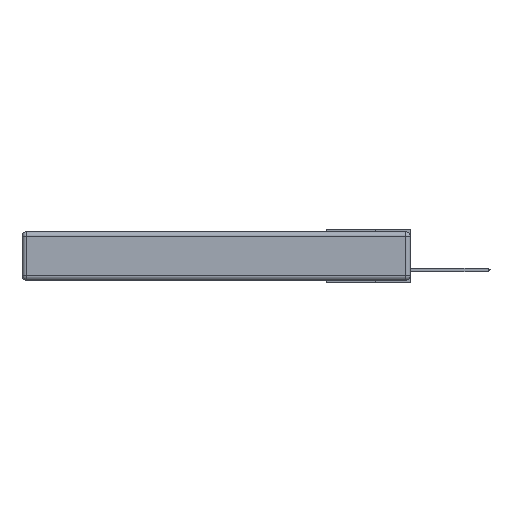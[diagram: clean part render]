
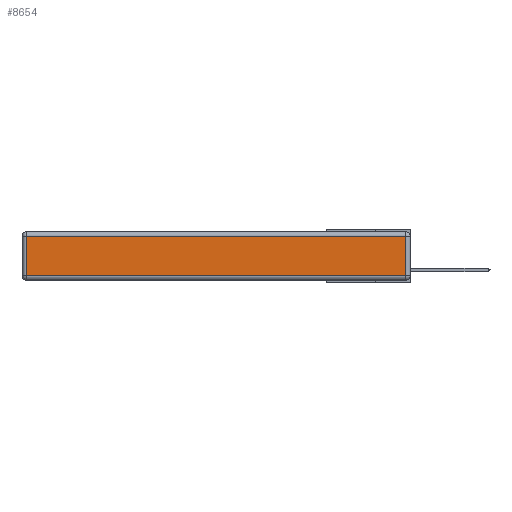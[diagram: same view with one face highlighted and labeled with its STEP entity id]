
A CAD part, left-side view. The second image highlights one B-rep face of the part: STEP entity #8654.
In plain terms, the highlighted planar face has unit normal (-1, 0, 0).
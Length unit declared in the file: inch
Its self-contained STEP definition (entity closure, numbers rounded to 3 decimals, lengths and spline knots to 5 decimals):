
#48 = EDGE_LOOP ( 'NONE', ( #139, #10912, #9708, #8686 ) ) ;
#139 = ORIENTED_EDGE ( 'NONE', *, *, #14576, .T. ) ;
#140 = CARTESIAN_POINT ( 'NONE',  ( 0., 0.03, -0.313 ) ) ;
#1244 = CARTESIAN_POINT ( 'NONE',  ( 0., 2.72, -0.343 ) ) ;
#1302 = CARTESIAN_POINT ( 'NONE',  ( 0., 0.03, -0.03 ) ) ;
#1592 = PLANE ( 'NONE',  #11813 ) ;
#2971 = VECTOR ( 'NONE', #4222, 39.37008 ) ;
#3200 = CARTESIAN_POINT ( 'NONE',  ( 0., 2.72, -0.313 ) ) ;
#4019 = VERTEX_POINT ( 'NONE', #1302 ) ;
#4164 = CARTESIAN_POINT ( 'NONE',  ( 0., 0., -0.313 ) ) ;
#4222 = DIRECTION ( 'NONE',  ( 0., 0., 1. ) ) ;
#4518 = DIRECTION ( 'NONE',  ( 0., 0., 1. ) ) ;
#5435 = VECTOR ( 'NONE', #10893, 39.37008 ) ;
#5450 = CARTESIAN_POINT ( 'NONE',  ( 0., 0.03, -0.343 ) ) ;
#5702 = VECTOR ( 'NONE', #16272, 39.37008 ) ;
#6993 = LINE ( 'NONE', #5450, #2971 ) ;
#7163 = VECTOR ( 'NONE', #10068, 39.37008 ) ;
#7431 = VERTEX_POINT ( 'NONE', #140 ) ;
#8091 = EDGE_CURVE ( 'NONE', #4019, #15879, #12069, .T. ) ;
#8401 = EDGE_CURVE ( 'NONE', #7431, #4019, #6993, .T. ) ;
#8513 = VERTEX_POINT ( 'NONE', #3200 ) ;
#8654 = ADVANCED_FACE ( 'NONE', ( #8674 ), #1592, .T. ) ;
#8674 = FACE_OUTER_BOUND ( 'NONE', #48, .T. ) ;
#8686 = ORIENTED_EDGE ( 'NONE', *, *, #9237, .T. ) ;
#9237 = EDGE_CURVE ( 'NONE', #15879, #8513, #16405, .T. ) ;
#9708 = ORIENTED_EDGE ( 'NONE', *, *, #8091, .T. ) ;
#10068 = DIRECTION ( 'NONE',  ( 0., 0., -1. ) ) ;
#10893 = DIRECTION ( 'NONE',  ( 0., -1., 0. ) ) ;
#10912 = ORIENTED_EDGE ( 'NONE', *, *, #8401, .T. ) ;
#11434 = CARTESIAN_POINT ( 'NONE',  ( 0., 2.72, -0.03 ) ) ;
#11545 = CARTESIAN_POINT ( 'NONE',  ( 0., 0., -0.343 ) ) ;
#11813 = AXIS2_PLACEMENT_3D ( 'NONE', #11545, #12949, #4518 ) ;
#12069 = LINE ( 'NONE', #14879, #5702 ) ;
#12949 = DIRECTION ( 'NONE',  ( -1., 0., 0. ) ) ;
#13050 = LINE ( 'NONE', #4164, #5435 ) ;
#14576 = EDGE_CURVE ( 'NONE', #8513, #7431, #13050, .T. ) ;
#14879 = CARTESIAN_POINT ( 'NONE',  ( 0., 2.75, -0.03 ) ) ;
#15879 = VERTEX_POINT ( 'NONE', #11434 ) ;
#16272 = DIRECTION ( 'NONE',  ( 0., 1., 0. ) ) ;
#16405 = LINE ( 'NONE', #1244, #7163 ) ;
